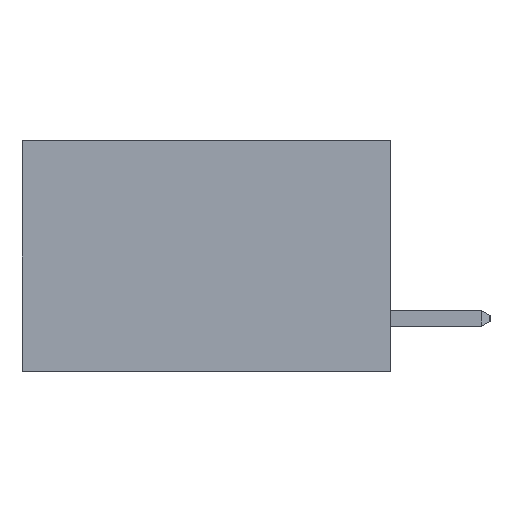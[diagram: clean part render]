
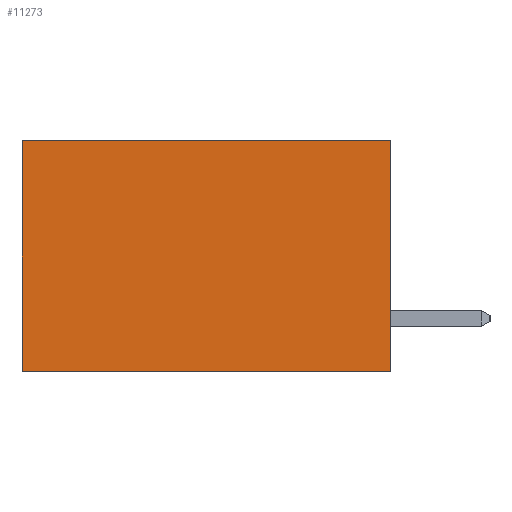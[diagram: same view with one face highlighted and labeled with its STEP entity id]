
A CAD part, left-side view. The second image highlights one B-rep face of the part: STEP entity #11273.
In plain terms, the highlighted planar face has unit normal (-1, 0, 0).
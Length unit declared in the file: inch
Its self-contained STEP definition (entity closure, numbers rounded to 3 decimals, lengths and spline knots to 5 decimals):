
#860 = VERTEX_POINT ( 'NONE', #9201 ) ;
#1000 = ORIENTED_EDGE ( 'NONE', *, *, #1761, .F. ) ;
#1074 = LINE ( 'NONE', #12742, #18258 ) ;
#1761 = EDGE_CURVE ( 'NONE', #14235, #3591, #1074, .T. ) ;
#2006 = EDGE_LOOP ( 'NONE', ( #9533, #2453, #1000, #10213 ) ) ;
#2109 = DIRECTION ( 'NONE',  ( 0., 1., 0. ) ) ;
#2231 = LINE ( 'NONE', #16710, #3787 ) ;
#2453 = ORIENTED_EDGE ( 'NONE', *, *, #11764, .F. ) ;
#3297 = LINE ( 'NONE', #8798, #19897 ) ;
#3591 = VERTEX_POINT ( 'NONE', #18148 ) ;
#3787 = VECTOR ( 'NONE', #8358, 39.37008 ) ;
#4147 = DIRECTION ( 'NONE',  ( 1., 0., 0. ) ) ;
#7026 = CARTESIAN_POINT ( 'NONE',  ( 0.277, 0., -0.37 ) ) ;
#8358 = DIRECTION ( 'NONE',  ( 0., 0., -1. ) ) ;
#8788 = FACE_OUTER_BOUND ( 'NONE', #2006, .T. ) ;
#8798 = CARTESIAN_POINT ( 'NONE',  ( 0.277, 0., 0. ) ) ;
#9201 = CARTESIAN_POINT ( 'NONE',  ( 0.277, 0.59, 0. ) ) ;
#9533 = ORIENTED_EDGE ( 'NONE', *, *, #13381, .T. ) ;
#10213 = ORIENTED_EDGE ( 'NONE', *, *, #11802, .T. ) ;
#11273 = ADVANCED_FACE ( 'NONE', ( #8788 ), #20666, .F. ) ;
#11764 = EDGE_CURVE ( 'NONE', #3591, #20893, #20897, .T. ) ;
#11802 = EDGE_CURVE ( 'NONE', #14235, #860, #3297, .T. ) ;
#12742 = CARTESIAN_POINT ( 'NONE',  ( 0.277, 0., -0.37 ) ) ;
#13381 = EDGE_CURVE ( 'NONE', #860, #20893, #2231, .T. ) ;
#14191 = CARTESIAN_POINT ( 'NONE',  ( 0.277, 0., -0.37 ) ) ;
#14235 = VERTEX_POINT ( 'NONE', #17107 ) ;
#15213 = CARTESIAN_POINT ( 'NONE',  ( 0.277, 0.59, -0.37 ) ) ;
#15857 = DIRECTION ( 'NONE',  ( 0., 0., -1. ) ) ;
#16702 = DIRECTION ( 'NONE',  ( 0., 0., -1. ) ) ;
#16710 = CARTESIAN_POINT ( 'NONE',  ( 0.277, 0.59, -0.37 ) ) ;
#17107 = CARTESIAN_POINT ( 'NONE',  ( 0.277, 0., 0. ) ) ;
#18148 = CARTESIAN_POINT ( 'NONE',  ( 0.277, 0., -0.37 ) ) ;
#18258 = VECTOR ( 'NONE', #16702, 39.37008 ) ;
#19585 = AXIS2_PLACEMENT_3D ( 'NONE', #14191, #4147, #15857 ) ;
#19897 = VECTOR ( 'NONE', #20356, 39.37008 ) ;
#20356 = DIRECTION ( 'NONE',  ( 0., 1., 0. ) ) ;
#20401 = VECTOR ( 'NONE', #2109, 39.37008 ) ;
#20666 = PLANE ( 'NONE',  #19585 ) ;
#20893 = VERTEX_POINT ( 'NONE', #15213 ) ;
#20897 = LINE ( 'NONE', #7026, #20401 ) ;
